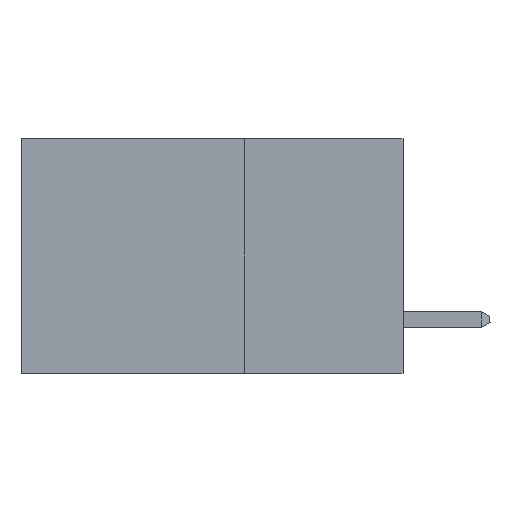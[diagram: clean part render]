
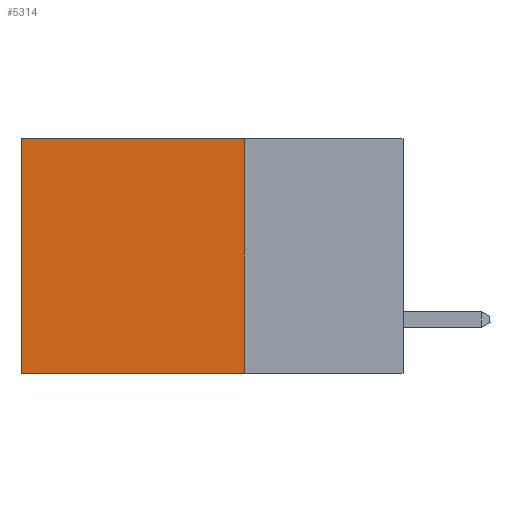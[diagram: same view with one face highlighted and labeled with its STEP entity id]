
A CAD part, left-side view. The second image highlights one B-rep face of the part: STEP entity #5314.
In plain terms, the highlighted planar face has unit normal (-1, 0, 0).
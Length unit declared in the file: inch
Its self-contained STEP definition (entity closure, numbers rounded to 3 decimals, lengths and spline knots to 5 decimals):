
#80 = VECTOR ( 'NONE', #8539, 39.37008 ) ;
#734 = DIRECTION ( 'NONE',  ( 1., 0., 0. ) ) ;
#1265 = VECTOR ( 'NONE', #2244, 39.37008 ) ;
#1665 = CARTESIAN_POINT ( 'NONE',  ( 0.2875, 0.25, -0.37 ) ) ;
#1673 = FACE_OUTER_BOUND ( 'NONE', #3918, .T. ) ;
#1947 = LINE ( 'NONE', #12590, #1265 ) ;
#2225 = VERTEX_POINT ( 'NONE', #12272 ) ;
#2244 = DIRECTION ( 'NONE',  ( 0., 0., -1. ) ) ;
#2453 = DIRECTION ( 'NONE',  ( 0., 0., -1. ) ) ;
#2883 = VECTOR ( 'NONE', #2453, 39.37008 ) ;
#3010 = VERTEX_POINT ( 'NONE', #3691 ) ;
#3065 = DIRECTION ( 'NONE',  ( 0., 0., -1. ) ) ;
#3201 = CARTESIAN_POINT ( 'NONE',  ( 0.2875, 0.25, 0. ) ) ;
#3263 = LINE ( 'NONE', #8330, #2883 ) ;
#3691 = CARTESIAN_POINT ( 'NONE',  ( 0.2875, 0.6, -0.37 ) ) ;
#3918 = EDGE_LOOP ( 'NONE', ( #8653, #8386, #12207, #10290 ) ) ;
#4319 = VERTEX_POINT ( 'NONE', #6770 ) ;
#4355 = EDGE_CURVE ( 'NONE', #4319, #11996, #4841, .T. ) ;
#4841 = LINE ( 'NONE', #3201, #13655 ) ;
#5079 = DIRECTION ( 'NONE',  ( 0., 1., 0. ) ) ;
#5314 = ADVANCED_FACE ( 'NONE', ( #1673 ), #6525, .F. ) ;
#6452 = EDGE_CURVE ( 'NONE', #2225, #3010, #14867, .T. ) ;
#6525 = PLANE ( 'NONE',  #14082 ) ;
#6770 = CARTESIAN_POINT ( 'NONE',  ( 0.2875, 0.25, 0. ) ) ;
#7686 = CARTESIAN_POINT ( 'NONE',  ( 0.2875, 0.25, 0. ) ) ;
#8330 = CARTESIAN_POINT ( 'NONE',  ( 0.2875, 0.6, 0. ) ) ;
#8386 = ORIENTED_EDGE ( 'NONE', *, *, #6452, .F. ) ;
#8539 = DIRECTION ( 'NONE',  ( 0., 1., 0. ) ) ;
#8653 = ORIENTED_EDGE ( 'NONE', *, *, #14599, .T. ) ;
#9066 = EDGE_CURVE ( 'NONE', #4319, #2225, #1947, .T. ) ;
#9722 = CARTESIAN_POINT ( 'NONE',  ( 0.2875, 0.6, 0. ) ) ;
#10290 = ORIENTED_EDGE ( 'NONE', *, *, #4355, .T. ) ;
#11996 = VERTEX_POINT ( 'NONE', #9722 ) ;
#12207 = ORIENTED_EDGE ( 'NONE', *, *, #9066, .F. ) ;
#12272 = CARTESIAN_POINT ( 'NONE',  ( 0.2875, 0.25, -0.37 ) ) ;
#12590 = CARTESIAN_POINT ( 'NONE',  ( 0.2875, 0.25, 0. ) ) ;
#13655 = VECTOR ( 'NONE', #5079, 39.37008 ) ;
#14082 = AXIS2_PLACEMENT_3D ( 'NONE', #7686, #734, #3065 ) ;
#14599 = EDGE_CURVE ( 'NONE', #11996, #3010, #3263, .T. ) ;
#14867 = LINE ( 'NONE', #1665, #80 ) ;
